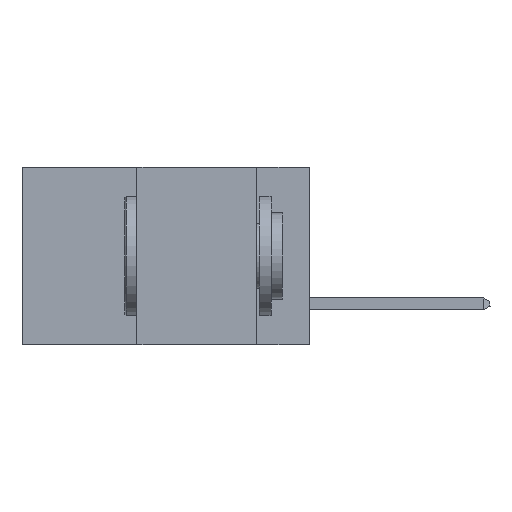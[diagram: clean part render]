
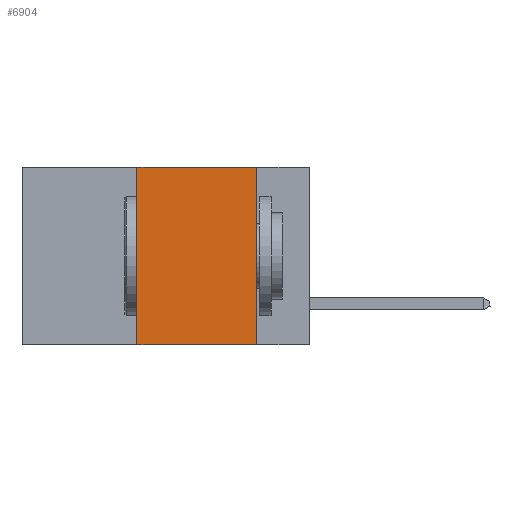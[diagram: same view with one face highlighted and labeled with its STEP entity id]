
A CAD part, left-side view. The second image highlights one B-rep face of the part: STEP entity #6904.
In plain terms, the highlighted planar face has unit normal (-1, 0, 0).
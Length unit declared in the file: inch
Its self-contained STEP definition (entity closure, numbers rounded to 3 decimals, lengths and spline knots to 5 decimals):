
#156 = CARTESIAN_POINT ( 'NONE',  ( 0., 0.36, -0.37 ) ) ;
#1862 = VERTEX_POINT ( 'NONE', #156 ) ;
#6881 = LINE ( 'NONE', #24034, #39139 ) ;
#6904 = ADVANCED_FACE ( 'NONE', ( #27541 ), #35467, .F. ) ;
#7342 = CARTESIAN_POINT ( 'NONE',  ( 0., 0.11, 0. ) ) ;
#7761 = ORIENTED_EDGE ( 'NONE', *, *, #31337, .T. ) ;
#8552 = DIRECTION ( 'NONE',  ( 0., 0., 1. ) ) ;
#8651 = VERTEX_POINT ( 'NONE', #7342 ) ;
#8652 = VECTOR ( 'NONE', #24048, 39.37008 ) ;
#8766 = VERTEX_POINT ( 'NONE', #14049 ) ;
#9921 = VECTOR ( 'NONE', #25619, 39.37008 ) ;
#10758 = CARTESIAN_POINT ( 'NONE',  ( 0., 0.6, -0.37 ) ) ;
#11262 = VECTOR ( 'NONE', #20323, 39.37008 ) ;
#13625 = VERTEX_POINT ( 'NONE', #28995 ) ;
#14049 = CARTESIAN_POINT ( 'NONE',  ( 0., 0.36, 0. ) ) ;
#16775 = DIRECTION ( 'NONE',  ( 1., 0., 0. ) ) ;
#20088 = CARTESIAN_POINT ( 'NONE',  ( 0., 0.6, 0. ) ) ;
#20167 = EDGE_CURVE ( 'NONE', #8651, #13625, #27700, .T. ) ;
#20323 = DIRECTION ( 'NONE',  ( 0., -1., 0. ) ) ;
#20842 = ORIENTED_EDGE ( 'NONE', *, *, #34535, .F. ) ;
#22627 = CARTESIAN_POINT ( 'NONE',  ( 0., 0.6, 0. ) ) ;
#23649 = LINE ( 'NONE', #22627, #9921 ) ;
#24034 = CARTESIAN_POINT ( 'NONE',  ( 0., 0.36, 0. ) ) ;
#24048 = DIRECTION ( 'NONE',  ( 0., 0., -1. ) ) ;
#25619 = DIRECTION ( 'NONE',  ( 0., -1., 0. ) ) ;
#27541 = FACE_OUTER_BOUND ( 'NONE', #39026, .T. ) ;
#27700 = LINE ( 'NONE', #33562, #8652 ) ;
#28687 = ORIENTED_EDGE ( 'NONE', *, *, #20167, .F. ) ;
#28995 = CARTESIAN_POINT ( 'NONE',  ( 0., 0.11, -0.37 ) ) ;
#31337 = EDGE_CURVE ( 'NONE', #1862, #13625, #37114, .T. ) ;
#33562 = CARTESIAN_POINT ( 'NONE',  ( 0., 0.11, 0. ) ) ;
#34535 = EDGE_CURVE ( 'NONE', #8766, #8651, #23649, .T. ) ;
#35361 = EDGE_CURVE ( 'NONE', #1862, #8766, #6881, .T. ) ;
#35467 = PLANE ( 'NONE',  #36198 ) ;
#36198 = AXIS2_PLACEMENT_3D ( 'NONE', #20088, #16775, #38608 ) ;
#36881 = ORIENTED_EDGE ( 'NONE', *, *, #35361, .F. ) ;
#37114 = LINE ( 'NONE', #10758, #11262 ) ;
#38608 = DIRECTION ( 'NONE',  ( 0., 0., -1. ) ) ;
#39026 = EDGE_LOOP ( 'NONE', ( #28687, #20842, #36881, #7761 ) ) ;
#39139 = VECTOR ( 'NONE', #8552, 39.37008 ) ;
